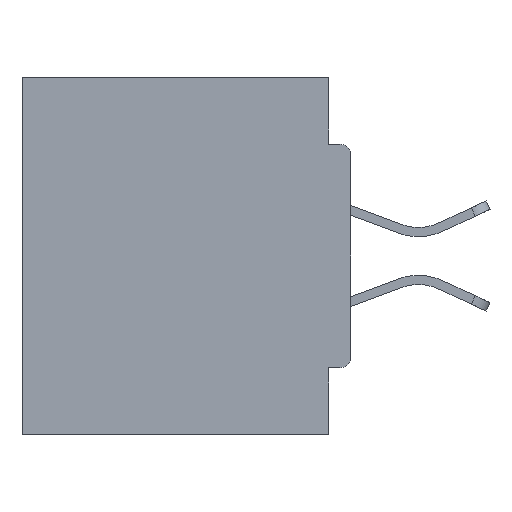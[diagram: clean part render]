
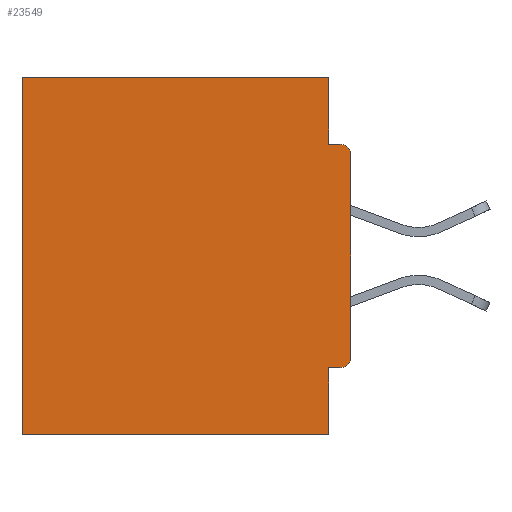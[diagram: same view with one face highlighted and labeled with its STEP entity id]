
A CAD part, left-side view. The second image highlights one B-rep face of the part: STEP entity #23549.
In plain terms, the highlighted planar face has unit normal (-1, 0, 0).
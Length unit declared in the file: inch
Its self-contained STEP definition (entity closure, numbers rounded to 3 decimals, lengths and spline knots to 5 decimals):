
#537 = CARTESIAN_POINT ( 'NONE',  ( 0.298, 0.46, 0. ) ) ;
#580 = ORIENTED_EDGE ( 'NONE', *, *, #3328, .T. ) ;
#1130 = ORIENTED_EDGE ( 'NONE', *, *, #11340, .F. ) ;
#1489 = CARTESIAN_POINT ( 'NONE',  ( 0.298, 0.031, -0.5 ) ) ;
#3328 = EDGE_CURVE ( 'NONE', #4592, #31853, #31301, .T. ) ;
#3428 = ORIENTED_EDGE ( 'NONE', *, *, #7903, .F. ) ;
#4592 = VERTEX_POINT ( 'NONE', #26878 ) ;
#4616 = CARTESIAN_POINT ( 'NONE',  ( 0.298, 0.031, 0. ) ) ;
#5684 = LINE ( 'NONE', #6518, #6691 ) ;
#5962 = DIRECTION ( 'NONE',  ( 0., 0., -1. ) ) ;
#6144 = DIRECTION ( 'NONE',  ( 0., 0., -1. ) ) ;
#6518 = CARTESIAN_POINT ( 'NONE',  ( 0.298, 0., 0. ) ) ;
#6561 = EDGE_CURVE ( 'NONE', #23338, #7130, #30637, .T. ) ;
#6626 = VERTEX_POINT ( 'NONE', #39177 ) ;
#6691 = VECTOR ( 'NONE', #13310, 39.37008 ) ;
#7130 = VERTEX_POINT ( 'NONE', #39241 ) ;
#7273 = VECTOR ( 'NONE', #25874, 39.37008 ) ;
#7441 = LINE ( 'NONE', #31826, #15333 ) ;
#7903 = EDGE_CURVE ( 'NONE', #4592, #6626, #17940, .T. ) ;
#8715 = ORIENTED_EDGE ( 'NONE', *, *, #17553, .F. ) ;
#8891 = VECTOR ( 'NONE', #34455, 39.37008 ) ;
#10141 = ORIENTED_EDGE ( 'NONE', *, *, #34005, .T. ) ;
#10455 = EDGE_CURVE ( 'NONE', #13353, #11497, #25032, .T. ) ;
#10763 = EDGE_CURVE ( 'NONE', #32418, #31853, #23085, .T. ) ;
#11340 = EDGE_CURVE ( 'NONE', #6626, #32756, #26426, .T. ) ;
#11497 = VERTEX_POINT ( 'NONE', #22015 ) ;
#11661 = CIRCLE ( 'NONE', #21427, 0.015 ) ;
#12188 = DIRECTION ( 'NONE',  ( -1., 0., 0. ) ) ;
#13073 = DIRECTION ( 'NONE',  ( -1., 0., 0. ) ) ;
#13239 = DIRECTION ( 'NONE',  ( 0., 0., -1. ) ) ;
#13310 = DIRECTION ( 'NONE',  ( 0., 1., 0. ) ) ;
#13353 = VERTEX_POINT ( 'NONE', #4616 ) ;
#13680 = AXIS2_PLACEMENT_3D ( 'NONE', #33842, #21407, #21134 ) ;
#14308 = VECTOR ( 'NONE', #37872, 39.37008 ) ;
#15333 = VECTOR ( 'NONE', #25643, 39.37008 ) ;
#15469 = VECTOR ( 'NONE', #13239, 39.37008 ) ;
#16516 = VECTOR ( 'NONE', #39146, 39.37008 ) ;
#16685 = CARTESIAN_POINT ( 'NONE',  ( 0.298, 0.031, -0.5 ) ) ;
#17553 = EDGE_CURVE ( 'NONE', #32756, #7130, #20021, .T. ) ;
#17940 = LINE ( 'NONE', #35682, #16516 ) ;
#20021 = LINE ( 'NONE', #29601, #7273 ) ;
#20508 = EDGE_CURVE ( 'NONE', #32418, #20925, #11661, .T. ) ;
#20925 = VERTEX_POINT ( 'NONE', #30238 ) ;
#21075 = ORIENTED_EDGE ( 'NONE', *, *, #40555, .F. ) ;
#21134 = DIRECTION ( 'NONE',  ( 0., 0., -1. ) ) ;
#21407 = DIRECTION ( 'NONE',  ( 1., 0., 0. ) ) ;
#21427 = AXIS2_PLACEMENT_3D ( 'NONE', #37155, #12188, #5962 ) ;
#22015 = CARTESIAN_POINT ( 'NONE',  ( 0.298, 0.031, -0.0935 ) ) ;
#22163 = CARTESIAN_POINT ( 'NONE',  ( 0.298, 0., 0. ) ) ;
#22325 = EDGE_LOOP ( 'NONE', ( #34925, #21075, #33676, #10141, #25047, #8715, #1130, #3428, #580, #35928 ) ) ;
#22509 = CARTESIAN_POINT ( 'NONE',  ( 0.298, 0., -0.3915 ) ) ;
#23085 = LINE ( 'NONE', #22163, #14308 ) ;
#23338 = VERTEX_POINT ( 'NONE', #537 ) ;
#23527 = VECTOR ( 'NONE', #35983, 39.37008 ) ;
#23549 = ADVANCED_FACE ( 'NONE', ( #24538 ), #40127, .F. ) ;
#24538 = FACE_OUTER_BOUND ( 'NONE', #22325, .T. ) ;
#25032 = LINE ( 'NONE', #31345, #8891 ) ;
#25047 = ORIENTED_EDGE ( 'NONE', *, *, #6561, .T. ) ;
#25643 = DIRECTION ( 'NONE',  ( 0., -1., 0. ) ) ;
#25874 = DIRECTION ( 'NONE',  ( 0., 1., 0. ) ) ;
#26426 = LINE ( 'NONE', #1489, #23527 ) ;
#26878 = CARTESIAN_POINT ( 'NONE',  ( 0.298, 0.015, -0.4065 ) ) ;
#28792 = CARTESIAN_POINT ( 'NONE',  ( 0.298, 0.46, 0. ) ) ;
#29601 = CARTESIAN_POINT ( 'NONE',  ( 0.298, 0., -0.5 ) ) ;
#30238 = CARTESIAN_POINT ( 'NONE',  ( 0.298, 0.015, -0.0935 ) ) ;
#30637 = LINE ( 'NONE', #28792, #15469 ) ;
#31301 = CIRCLE ( 'NONE', #34586, 0.015 ) ;
#31345 = CARTESIAN_POINT ( 'NONE',  ( 0.298, 0.031, -0.5 ) ) ;
#31791 = CARTESIAN_POINT ( 'NONE',  ( 0.298, 0.015, -0.3915 ) ) ;
#31826 = CARTESIAN_POINT ( 'NONE',  ( 0.298, 0., -0.0935 ) ) ;
#31853 = VERTEX_POINT ( 'NONE', #22509 ) ;
#32418 = VERTEX_POINT ( 'NONE', #37070 ) ;
#32756 = VERTEX_POINT ( 'NONE', #16685 ) ;
#33676 = ORIENTED_EDGE ( 'NONE', *, *, #10455, .F. ) ;
#33842 = CARTESIAN_POINT ( 'NONE',  ( 0.298, 0., 0. ) ) ;
#34005 = EDGE_CURVE ( 'NONE', #13353, #23338, #5684, .T. ) ;
#34455 = DIRECTION ( 'NONE',  ( 0., 0., -1. ) ) ;
#34586 = AXIS2_PLACEMENT_3D ( 'NONE', #31791, #13073, #6144 ) ;
#34925 = ORIENTED_EDGE ( 'NONE', *, *, #20508, .T. ) ;
#35682 = CARTESIAN_POINT ( 'NONE',  ( 0.298, 0., -0.4065 ) ) ;
#35928 = ORIENTED_EDGE ( 'NONE', *, *, #10763, .F. ) ;
#35983 = DIRECTION ( 'NONE',  ( 0., 0., -1. ) ) ;
#37070 = CARTESIAN_POINT ( 'NONE',  ( 0.298, 0., -0.1085 ) ) ;
#37155 = CARTESIAN_POINT ( 'NONE',  ( 0.298, 0.015, -0.1085 ) ) ;
#37872 = DIRECTION ( 'NONE',  ( 0., 0., -1. ) ) ;
#39146 = DIRECTION ( 'NONE',  ( 0., 1., 0. ) ) ;
#39177 = CARTESIAN_POINT ( 'NONE',  ( 0.298, 0.031, -0.4065 ) ) ;
#39241 = CARTESIAN_POINT ( 'NONE',  ( 0.298, 0.46, -0.5 ) ) ;
#40127 = PLANE ( 'NONE',  #13680 ) ;
#40555 = EDGE_CURVE ( 'NONE', #11497, #20925, #7441, .T. ) ;
